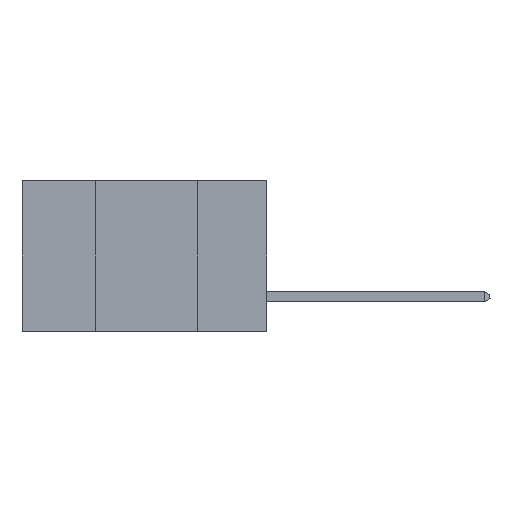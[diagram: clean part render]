
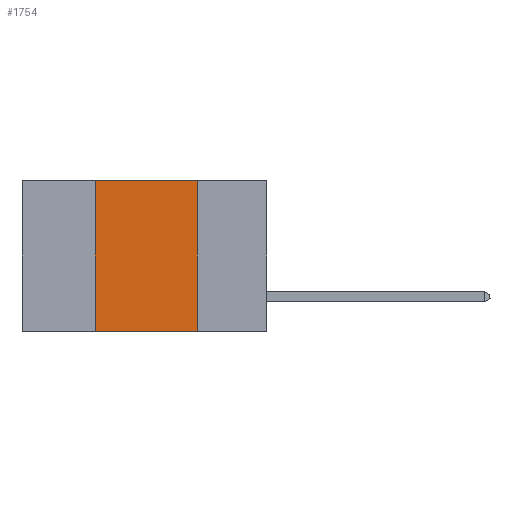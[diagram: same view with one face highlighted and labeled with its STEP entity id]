
A CAD part, left-side view. The second image highlights one B-rep face of the part: STEP entity #1754.
In plain terms, the highlighted planar face has unit normal (-1, 0, 0).
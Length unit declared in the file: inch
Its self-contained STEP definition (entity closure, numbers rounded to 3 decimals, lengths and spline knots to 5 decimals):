
#148 = AXIS2_PLACEMENT_3D ( 'NONE', #8320, #4054, #1781 ) ;
#1754 = ADVANCED_FACE ( 'NONE', ( #17238 ), #6336, .F. ) ;
#1781 = DIRECTION ( 'NONE',  ( 0., 0., -1. ) ) ;
#1935 = DIRECTION ( 'NONE',  ( 0., 0., -1. ) ) ;
#2737 = LINE ( 'NONE', #10227, #4864 ) ;
#2937 = EDGE_CURVE ( 'NONE', #15870, #20626, #16118, .T. ) ;
#3227 = EDGE_CURVE ( 'NONE', #20626, #22917, #18912, .T. ) ;
#4054 = DIRECTION ( 'NONE',  ( 1., 0., 0. ) ) ;
#4296 = CARTESIAN_POINT ( 'NONE',  ( 0., 0.17, 0. ) ) ;
#4381 = LINE ( 'NONE', #4296, #11151 ) ;
#4864 = VECTOR ( 'NONE', #12370, 39.37008 ) ;
#5129 = VECTOR ( 'NONE', #23133, 39.37008 ) ;
#5736 = ORIENTED_EDGE ( 'NONE', *, *, #13919, .F. ) ;
#6336 = PLANE ( 'NONE',  #148 ) ;
#8320 = CARTESIAN_POINT ( 'NONE',  ( 0., 0.6, 0. ) ) ;
#9935 = CARTESIAN_POINT ( 'NONE',  ( 0., 0.17, 0. ) ) ;
#9957 = ORIENTED_EDGE ( 'NONE', *, *, #3227, .F. ) ;
#10058 = VERTEX_POINT ( 'NONE', #13066 ) ;
#10227 = CARTESIAN_POINT ( 'NONE',  ( 0., 0.6, -0.37 ) ) ;
#10920 = CARTESIAN_POINT ( 'NONE',  ( 0., 0.42, 0. ) ) ;
#11151 = VECTOR ( 'NONE', #1935, 39.37008 ) ;
#11672 = CARTESIAN_POINT ( 'NONE',  ( 0., 0.42, -0.37 ) ) ;
#12370 = DIRECTION ( 'NONE',  ( 0., -1., 0. ) ) ;
#13066 = CARTESIAN_POINT ( 'NONE',  ( 0., 0.17, -0.37 ) ) ;
#13919 = EDGE_CURVE ( 'NONE', #22917, #10058, #4381, .T. ) ;
#14183 = EDGE_LOOP ( 'NONE', ( #5736, #9957, #22313, #27782 ) ) ;
#15870 = VERTEX_POINT ( 'NONE', #11672 ) ;
#16118 = LINE ( 'NONE', #26220, #19295 ) ;
#17238 = FACE_OUTER_BOUND ( 'NONE', #14183, .T. ) ;
#18043 = EDGE_CURVE ( 'NONE', #15870, #10058, #2737, .T. ) ;
#18912 = LINE ( 'NONE', #25203, #5129 ) ;
#19295 = VECTOR ( 'NONE', #26412, 39.37008 ) ;
#20626 = VERTEX_POINT ( 'NONE', #10920 ) ;
#22313 = ORIENTED_EDGE ( 'NONE', *, *, #2937, .F. ) ;
#22917 = VERTEX_POINT ( 'NONE', #9935 ) ;
#23133 = DIRECTION ( 'NONE',  ( 0., -1., 0. ) ) ;
#25203 = CARTESIAN_POINT ( 'NONE',  ( 0., 0.6, 0. ) ) ;
#26220 = CARTESIAN_POINT ( 'NONE',  ( 0., 0.42, 0. ) ) ;
#26412 = DIRECTION ( 'NONE',  ( 0., 0., 1. ) ) ;
#27782 = ORIENTED_EDGE ( 'NONE', *, *, #18043, .T. ) ;
